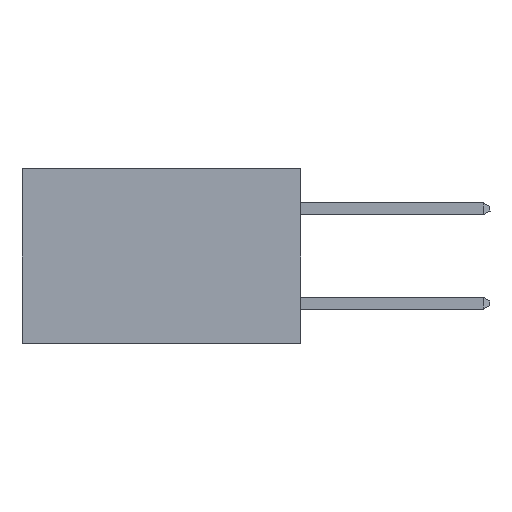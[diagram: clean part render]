
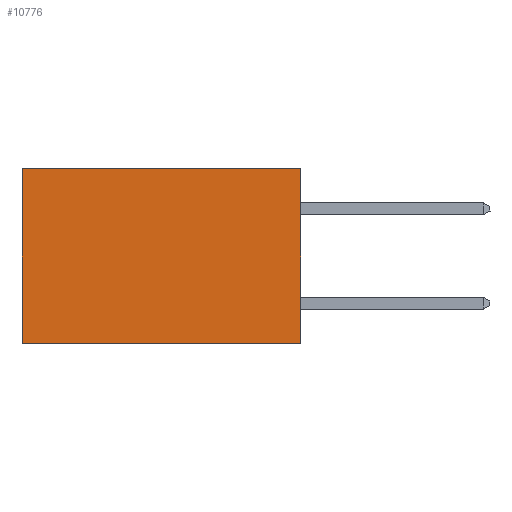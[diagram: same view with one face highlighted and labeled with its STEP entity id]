
A CAD part, left-side view. The second image highlights one B-rep face of the part: STEP entity #10776.
In plain terms, the highlighted planar face has unit normal (-1, 0, 0).
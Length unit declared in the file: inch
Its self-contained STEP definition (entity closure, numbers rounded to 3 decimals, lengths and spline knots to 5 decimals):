
#360 = DIRECTION ( 'NONE',  ( 1., 0., 0. ) ) ;
#768 = CARTESIAN_POINT ( 'NONE',  ( 0.277, 0., 0. ) ) ;
#932 = DIRECTION ( 'NONE',  ( 0., 1., 0. ) ) ;
#1739 = VERTEX_POINT ( 'NONE', #5310 ) ;
#3423 = LINE ( 'NONE', #768, #20128 ) ;
#3562 = AXIS2_PLACEMENT_3D ( 'NONE', #7673, #360, #13017 ) ;
#4842 = FACE_OUTER_BOUND ( 'NONE', #10897, .T. ) ;
#5072 = CARTESIAN_POINT ( 'NONE',  ( 0.277, 0.59, 0. ) ) ;
#5310 = CARTESIAN_POINT ( 'NONE',  ( 0.277, 0., -0.37 ) ) ;
#5375 = EDGE_CURVE ( 'NONE', #10507, #10633, #22194, .T. ) ;
#6141 = EDGE_CURVE ( 'NONE', #10367, #1739, #11160, .T. ) ;
#6236 = ORIENTED_EDGE ( 'NONE', *, *, #16698, .F. ) ;
#7673 = CARTESIAN_POINT ( 'NONE',  ( 0.277, 0., -0.37 ) ) ;
#8065 = CARTESIAN_POINT ( 'NONE',  ( 0.277, 0., -0.37 ) ) ;
#10329 = EDGE_CURVE ( 'NONE', #10367, #10507, #3423, .T. ) ;
#10367 = VERTEX_POINT ( 'NONE', #20541 ) ;
#10507 = VERTEX_POINT ( 'NONE', #5072 ) ;
#10633 = VERTEX_POINT ( 'NONE', #21307 ) ;
#10776 = ADVANCED_FACE ( 'NONE', ( #4842 ), #11229, .F. ) ;
#10897 = EDGE_LOOP ( 'NONE', ( #22459, #6236, #16316, #18862 ) ) ;
#11160 = LINE ( 'NONE', #8065, #19975 ) ;
#11229 = PLANE ( 'NONE',  #3562 ) ;
#12861 = VECTOR ( 'NONE', #16484, 39.37008 ) ;
#13017 = DIRECTION ( 'NONE',  ( 0., 0., -1. ) ) ;
#15977 = CARTESIAN_POINT ( 'NONE',  ( 0.277, 0.59, -0.37 ) ) ;
#16316 = ORIENTED_EDGE ( 'NONE', *, *, #6141, .F. ) ;
#16368 = VECTOR ( 'NONE', #932, 39.37008 ) ;
#16484 = DIRECTION ( 'NONE',  ( 0., 0., -1. ) ) ;
#16698 = EDGE_CURVE ( 'NONE', #1739, #10633, #21033, .T. ) ;
#16963 = DIRECTION ( 'NONE',  ( 0., 1., 0. ) ) ;
#18643 = DIRECTION ( 'NONE',  ( 0., 0., -1. ) ) ;
#18862 = ORIENTED_EDGE ( 'NONE', *, *, #10329, .T. ) ;
#19975 = VECTOR ( 'NONE', #18643, 39.37008 ) ;
#20128 = VECTOR ( 'NONE', #16963, 39.37008 ) ;
#20541 = CARTESIAN_POINT ( 'NONE',  ( 0.277, 0., 0. ) ) ;
#20549 = CARTESIAN_POINT ( 'NONE',  ( 0.277, 0., -0.37 ) ) ;
#21033 = LINE ( 'NONE', #20549, #16368 ) ;
#21307 = CARTESIAN_POINT ( 'NONE',  ( 0.277, 0.59, -0.37 ) ) ;
#22194 = LINE ( 'NONE', #15977, #12861 ) ;
#22459 = ORIENTED_EDGE ( 'NONE', *, *, #5375, .T. ) ;
